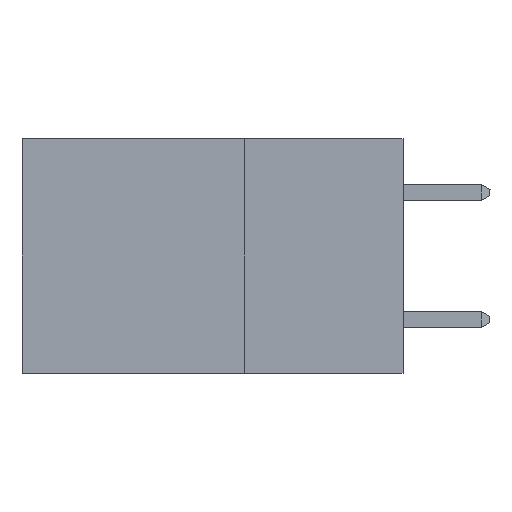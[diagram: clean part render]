
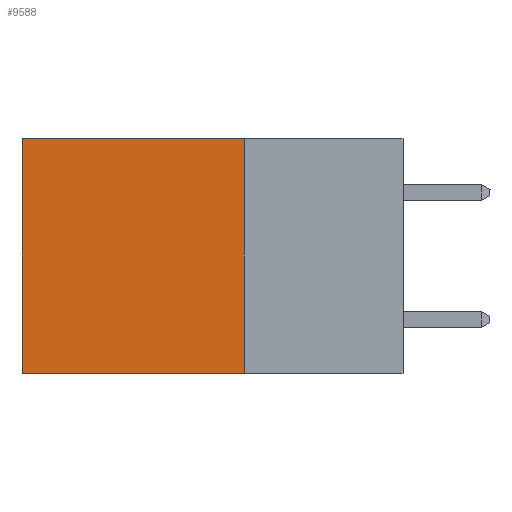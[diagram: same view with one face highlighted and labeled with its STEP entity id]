
A CAD part, left-side view. The second image highlights one B-rep face of the part: STEP entity #9588.
In plain terms, the highlighted planar face has unit normal (-1, 0, 0).
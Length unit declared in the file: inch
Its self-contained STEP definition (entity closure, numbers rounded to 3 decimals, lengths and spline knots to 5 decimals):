
#1539 = VECTOR ( 'NONE', #7365, 39.37008 ) ;
#1828 = AXIS2_PLACEMENT_3D ( 'NONE', #2622, #21168, #16844 ) ;
#2228 = EDGE_CURVE ( 'NONE', #19565, #11014, #10646, .T. ) ;
#2618 = EDGE_CURVE ( 'NONE', #9754, #17468, #16988, .T. ) ;
#2622 = CARTESIAN_POINT ( 'NONE',  ( 0.2875, 0.25, 0. ) ) ;
#3471 = LINE ( 'NONE', #4904, #4362 ) ;
#4362 = VECTOR ( 'NONE', #24410, 39.37008 ) ;
#4486 = CARTESIAN_POINT ( 'NONE',  ( 0.2875, 0.6, 0. ) ) ;
#4888 = VECTOR ( 'NONE', #9449, 39.37008 ) ;
#4904 = CARTESIAN_POINT ( 'NONE',  ( 0.2875, 0.25, -0.37 ) ) ;
#5382 = CARTESIAN_POINT ( 'NONE',  ( 0.2875, 0.25, 0. ) ) ;
#6361 = CARTESIAN_POINT ( 'NONE',  ( 0.2875, 0.25, -0.37 ) ) ;
#6460 = ORIENTED_EDGE ( 'NONE', *, *, #2228, .F. ) ;
#6944 = PLANE ( 'NONE',  #1828 ) ;
#7365 = DIRECTION ( 'NONE',  ( 0., 1., 0. ) ) ;
#8455 = DIRECTION ( 'NONE',  ( 0., 0., -1. ) ) ;
#9081 = LINE ( 'NONE', #5382, #1539 ) ;
#9266 = CARTESIAN_POINT ( 'NONE',  ( 0.2875, 0.25, 0. ) ) ;
#9449 = DIRECTION ( 'NONE',  ( 0., 0., -1. ) ) ;
#9588 = ADVANCED_FACE ( 'NONE', ( #23178 ), #6944, .F. ) ;
#9754 = VERTEX_POINT ( 'NONE', #19779 ) ;
#10646 = LINE ( 'NONE', #22552, #4888 ) ;
#10726 = ORIENTED_EDGE ( 'NONE', *, *, #2618, .T. ) ;
#11014 = VERTEX_POINT ( 'NONE', #6361 ) ;
#11871 = ORIENTED_EDGE ( 'NONE', *, *, #16793, .F. ) ;
#14122 = EDGE_CURVE ( 'NONE', #19565, #9754, #9081, .T. ) ;
#15867 = EDGE_LOOP ( 'NONE', ( #10726, #11871, #6460, #22281 ) ) ;
#16359 = VECTOR ( 'NONE', #8455, 39.37008 ) ;
#16793 = EDGE_CURVE ( 'NONE', #11014, #17468, #3471, .T. ) ;
#16844 = DIRECTION ( 'NONE',  ( 0., 0., -1. ) ) ;
#16988 = LINE ( 'NONE', #4486, #16359 ) ;
#17468 = VERTEX_POINT ( 'NONE', #18245 ) ;
#18245 = CARTESIAN_POINT ( 'NONE',  ( 0.2875, 0.6, -0.37 ) ) ;
#19565 = VERTEX_POINT ( 'NONE', #9266 ) ;
#19779 = CARTESIAN_POINT ( 'NONE',  ( 0.2875, 0.6, 0. ) ) ;
#21168 = DIRECTION ( 'NONE',  ( 1., 0., 0. ) ) ;
#22281 = ORIENTED_EDGE ( 'NONE', *, *, #14122, .T. ) ;
#22552 = CARTESIAN_POINT ( 'NONE',  ( 0.2875, 0.25, 0. ) ) ;
#23178 = FACE_OUTER_BOUND ( 'NONE', #15867, .T. ) ;
#24410 = DIRECTION ( 'NONE',  ( 0., 1., 0. ) ) ;
